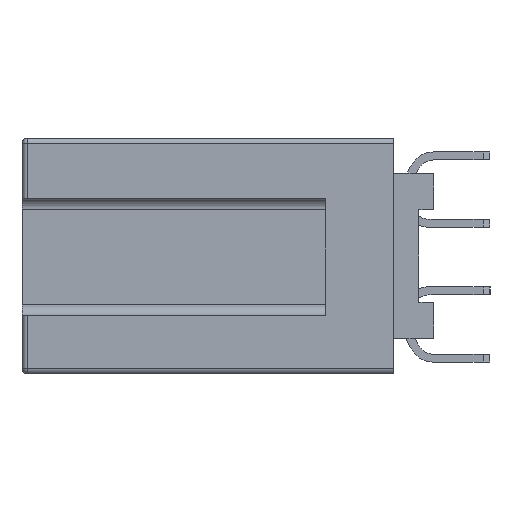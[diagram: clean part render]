
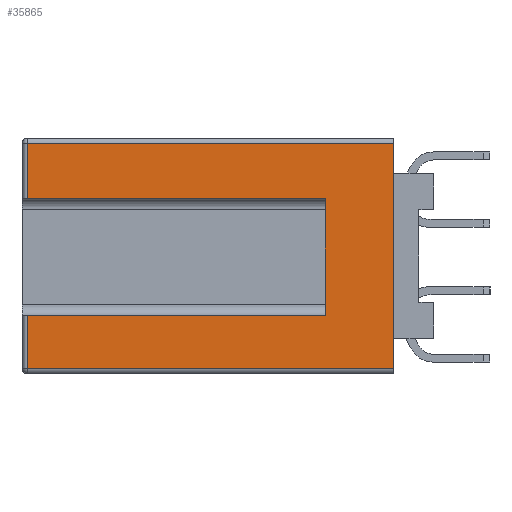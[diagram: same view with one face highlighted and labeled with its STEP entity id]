
A CAD part, left-side view. The second image highlights one B-rep face of the part: STEP entity #35865.
In plain terms, the highlighted planar face has unit normal (-1, 0, 0).
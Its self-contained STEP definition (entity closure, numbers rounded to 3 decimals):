
#1262 = LINE ( 'NONE', #18736, #18090 ) ;
#1879 = CARTESIAN_POINT ( 'NONE',  ( 0., 15.3, -6.68 ) ) ;
#2008 = VERTEX_POINT ( 'NONE', #27149 ) ;
#2173 = DIRECTION ( 'NONE',  ( 0., 0., -1. ) ) ;
#2955 = VECTOR ( 'NONE', #10521, 1000. ) ;
#3433 = EDGE_CURVE ( 'NONE', #19545, #24952, #4010, .T. ) ;
#3964 = FACE_OUTER_BOUND ( 'NONE', #7352, .T. ) ;
#4010 = LINE ( 'NONE', #17216, #2955 ) ;
#6409 = VECTOR ( 'NONE', #2173, 1000. ) ;
#6799 = LINE ( 'NONE', #23446, #11409 ) ;
#7003 = CARTESIAN_POINT ( 'NONE',  ( 0., 1.5, -0.2 ) ) ;
#7352 = EDGE_LOOP ( 'NONE', ( #27464, #27074, #8213, #27285, #31900, #20598, #10244, #30862 ) ) ;
#7372 = DIRECTION ( 'NONE',  ( 0., -1., 0. ) ) ;
#8038 = DIRECTION ( 'NONE',  ( 0., 0., -1. ) ) ;
#8213 = ORIENTED_EDGE ( 'NONE', *, *, #3433, .F. ) ;
#8794 = CARTESIAN_POINT ( 'NONE',  ( 0., 4.07, -6.68 ) ) ;
#10056 = PLANE ( 'NONE',  #18334 ) ;
#10244 = ORIENTED_EDGE ( 'NONE', *, *, #36863, .T. ) ;
#10471 = CARTESIAN_POINT ( 'NONE',  ( 0., 15.5, 0. ) ) ;
#10521 = DIRECTION ( 'NONE',  ( 0., 0., -1. ) ) ;
#10623 = CARTESIAN_POINT ( 'NONE',  ( 0., 15.5, -8.68 ) ) ;
#11051 = DIRECTION ( 'NONE',  ( 0., 1., 0. ) ) ;
#11409 = VECTOR ( 'NONE', #8038, 1000. ) ;
#11878 = CARTESIAN_POINT ( 'NONE',  ( 0., 4.07, -2.28 ) ) ;
#13258 = VECTOR ( 'NONE', #29515, 1000. ) ;
#13833 = VERTEX_POINT ( 'NONE', #1879 ) ;
#14588 = CARTESIAN_POINT ( 'NONE',  ( 0., 15.3, -0.2 ) ) ;
#15171 = LINE ( 'NONE', #18846, #6409 ) ;
#15272 = CARTESIAN_POINT ( 'NONE',  ( 0., 4.07, -6.68 ) ) ;
#15734 = VECTOR ( 'NONE', #11051, 1000. ) ;
#16959 = DIRECTION ( 'NONE',  ( 0., 0., -1. ) ) ;
#17170 = DIRECTION ( 'NONE',  ( 1., 0., 0. ) ) ;
#17216 = CARTESIAN_POINT ( 'NONE',  ( 0., 1.5, 0. ) ) ;
#17817 = EDGE_CURVE ( 'NONE', #2008, #24952, #27042, .T. ) ;
#18090 = VECTOR ( 'NONE', #34340, 1000. ) ;
#18334 = AXIS2_PLACEMENT_3D ( 'NONE', #10471, #17170, #16959 ) ;
#18736 = CARTESIAN_POINT ( 'NONE',  ( 0., 4.07, -2.28 ) ) ;
#18846 = CARTESIAN_POINT ( 'NONE',  ( 0., 15.3, 0. ) ) ;
#19545 = VERTEX_POINT ( 'NONE', #7003 ) ;
#19788 = LINE ( 'NONE', #22819, #13258 ) ;
#20161 = CARTESIAN_POINT ( 'NONE',  ( 0., 15.3, -2.28 ) ) ;
#20563 = CARTESIAN_POINT ( 'NONE',  ( 0., 15.5, -0.2 ) ) ;
#20598 = ORIENTED_EDGE ( 'NONE', *, *, #29110, .T. ) ;
#21316 = VERTEX_POINT ( 'NONE', #15272 ) ;
#21595 = EDGE_CURVE ( 'NONE', #13833, #2008, #6799, .T. ) ;
#22819 = CARTESIAN_POINT ( 'NONE',  ( 0., 4.07, -2.28 ) ) ;
#23335 = VECTOR ( 'NONE', #7372, 1000. ) ;
#23446 = CARTESIAN_POINT ( 'NONE',  ( 0., 15.3, 0. ) ) ;
#24381 = EDGE_CURVE ( 'NONE', #19545, #30420, #27040, .T. ) ;
#24952 = VERTEX_POINT ( 'NONE', #38228 ) ;
#25917 = VECTOR ( 'NONE', #28670, 1000. ) ;
#27040 = LINE ( 'NONE', #20563, #15734 ) ;
#27042 = LINE ( 'NONE', #10623, #23335 ) ;
#27074 = ORIENTED_EDGE ( 'NONE', *, *, #17817, .T. ) ;
#27149 = CARTESIAN_POINT ( 'NONE',  ( 0., 15.3, -8.68 ) ) ;
#27285 = ORIENTED_EDGE ( 'NONE', *, *, #24381, .T. ) ;
#27464 = ORIENTED_EDGE ( 'NONE', *, *, #21595, .T. ) ;
#28245 = LINE ( 'NONE', #8794, #25917 ) ;
#28558 = VERTEX_POINT ( 'NONE', #11878 ) ;
#28670 = DIRECTION ( 'NONE',  ( 0., 1., 0. ) ) ;
#29110 = EDGE_CURVE ( 'NONE', #32304, #28558, #19788, .T. ) ;
#29515 = DIRECTION ( 'NONE',  ( 0., -1., 0. ) ) ;
#30420 = VERTEX_POINT ( 'NONE', #14588 ) ;
#30862 = ORIENTED_EDGE ( 'NONE', *, *, #35584, .T. ) ;
#31900 = ORIENTED_EDGE ( 'NONE', *, *, #39416, .T. ) ;
#32304 = VERTEX_POINT ( 'NONE', #20161 ) ;
#34340 = DIRECTION ( 'NONE',  ( 0., 0., -1. ) ) ;
#35584 = EDGE_CURVE ( 'NONE', #21316, #13833, #28245, .T. ) ;
#35865 = ADVANCED_FACE ( 'NONE', ( #3964 ), #10056, .F. ) ;
#36863 = EDGE_CURVE ( 'NONE', #28558, #21316, #1262, .T. ) ;
#38228 = CARTESIAN_POINT ( 'NONE',  ( 0., 1.5, -8.68 ) ) ;
#39416 = EDGE_CURVE ( 'NONE', #30420, #32304, #15171, .T. ) ;
